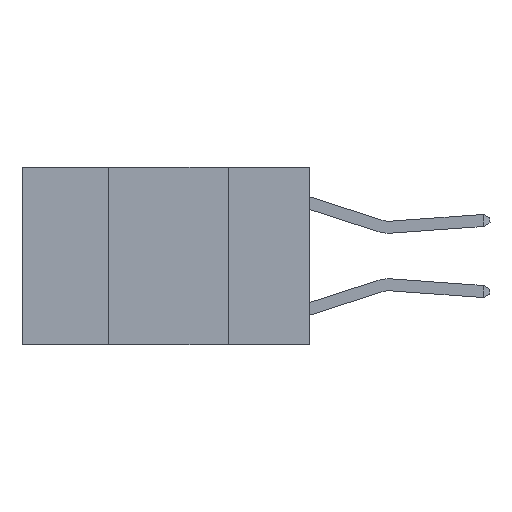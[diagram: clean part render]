
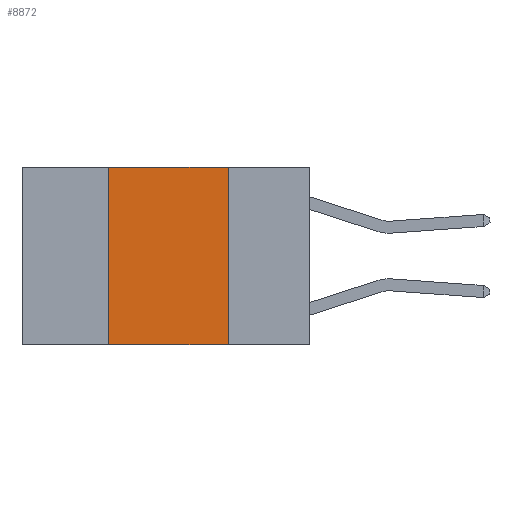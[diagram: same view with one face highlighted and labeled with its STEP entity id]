
A CAD part, left-side view. The second image highlights one B-rep face of the part: STEP entity #8872.
In plain terms, the highlighted planar face has unit normal (-1, 0, 0).
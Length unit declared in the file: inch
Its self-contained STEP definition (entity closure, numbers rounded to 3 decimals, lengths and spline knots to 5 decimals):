
#28 = DIRECTION ( 'NONE',  ( 0., 0., -1. ) ) ;
#283 = LINE ( 'NONE', #6997, #7839 ) ;
#519 = VERTEX_POINT ( 'NONE', #18685 ) ;
#869 = VECTOR ( 'NONE', #1934, 39.37008 ) ;
#1934 = DIRECTION ( 'NONE',  ( 0., -1., 0. ) ) ;
#2023 = ORIENTED_EDGE ( 'NONE', *, *, #14478, .F. ) ;
#2151 = VECTOR ( 'NONE', #10208, 39.37008 ) ;
#4027 = VERTEX_POINT ( 'NONE', #7190 ) ;
#4363 = VERTEX_POINT ( 'NONE', #19586 ) ;
#4799 = CARTESIAN_POINT ( 'NONE',  ( 0., 0.6, 0. ) ) ;
#5657 = FACE_OUTER_BOUND ( 'NONE', #15160, .T. ) ;
#6024 = VECTOR ( 'NONE', #17367, 39.37008 ) ;
#6245 = ORIENTED_EDGE ( 'NONE', *, *, #19575, .F. ) ;
#6997 = CARTESIAN_POINT ( 'NONE',  ( 0., 0.6, 0. ) ) ;
#7047 = LINE ( 'NONE', #14202, #6024 ) ;
#7190 = CARTESIAN_POINT ( 'NONE',  ( 0., 0.17, 0. ) ) ;
#7839 = VECTOR ( 'NONE', #18355, 39.37008 ) ;
#8051 = PLANE ( 'NONE',  #18738 ) ;
#8072 = VERTEX_POINT ( 'NONE', #20735 ) ;
#8872 = ADVANCED_FACE ( 'NONE', ( #5657 ), #8051, .F. ) ;
#9649 = DIRECTION ( 'NONE',  ( 1., 0., 0. ) ) ;
#10208 = DIRECTION ( 'NONE',  ( 0., 0., 1. ) ) ;
#11558 = CARTESIAN_POINT ( 'NONE',  ( 0., 0.6, -0.37 ) ) ;
#13722 = LINE ( 'NONE', #11558, #869 ) ;
#13858 = ORIENTED_EDGE ( 'NONE', *, *, #14798, .F. ) ;
#14202 = CARTESIAN_POINT ( 'NONE',  ( 0., 0.17, 0. ) ) ;
#14478 = EDGE_CURVE ( 'NONE', #4363, #4027, #283, .T. ) ;
#14798 = EDGE_CURVE ( 'NONE', #4027, #519, #7047, .T. ) ;
#15160 = EDGE_LOOP ( 'NONE', ( #13858, #2023, #6245, #19195 ) ) ;
#15505 = LINE ( 'NONE', #18301, #2151 ) ;
#17367 = DIRECTION ( 'NONE',  ( 0., 0., -1. ) ) ;
#18301 = CARTESIAN_POINT ( 'NONE',  ( 0., 0.42, 0. ) ) ;
#18355 = DIRECTION ( 'NONE',  ( 0., -1., 0. ) ) ;
#18685 = CARTESIAN_POINT ( 'NONE',  ( 0., 0.17, -0.37 ) ) ;
#18738 = AXIS2_PLACEMENT_3D ( 'NONE', #4799, #9649, #28 ) ;
#19195 = ORIENTED_EDGE ( 'NONE', *, *, #19485, .T. ) ;
#19485 = EDGE_CURVE ( 'NONE', #8072, #519, #13722, .T. ) ;
#19575 = EDGE_CURVE ( 'NONE', #8072, #4363, #15505, .T. ) ;
#19586 = CARTESIAN_POINT ( 'NONE',  ( 0., 0.42, 0. ) ) ;
#20735 = CARTESIAN_POINT ( 'NONE',  ( 0., 0.42, -0.37 ) ) ;
